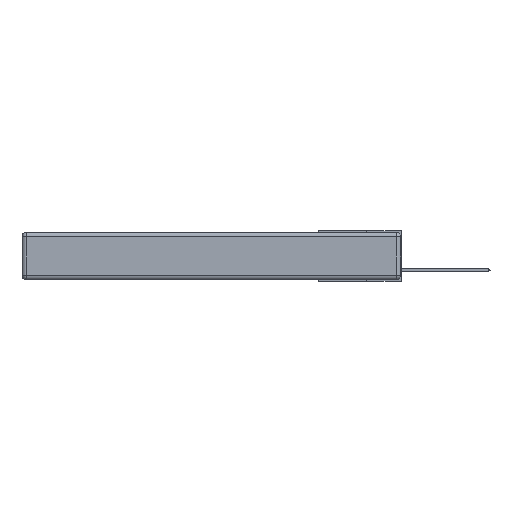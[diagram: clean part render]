
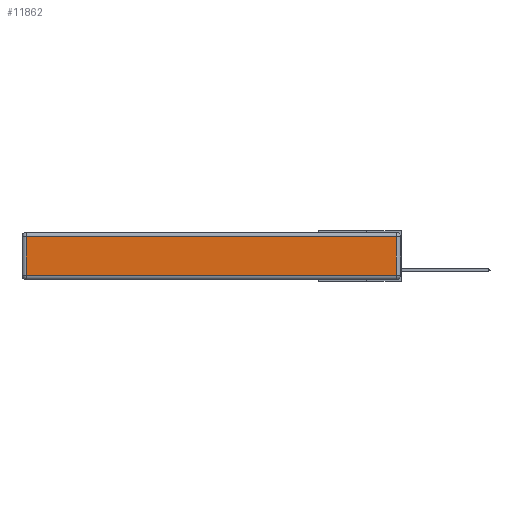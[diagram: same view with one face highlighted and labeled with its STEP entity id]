
A CAD part, left-side view. The second image highlights one B-rep face of the part: STEP entity #11862.
In plain terms, the highlighted planar face has unit normal (-1, 0, 0).
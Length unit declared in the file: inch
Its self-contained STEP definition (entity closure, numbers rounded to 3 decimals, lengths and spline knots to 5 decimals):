
#286 = CARTESIAN_POINT ( 'NONE',  ( 0., 2.72, -0.313 ) ) ;
#746 = CARTESIAN_POINT ( 'NONE',  ( 0., 0.03, -0.03 ) ) ;
#1514 = VECTOR ( 'NONE', #6466, 39.37008 ) ;
#2364 = VECTOR ( 'NONE', #9813, 39.37008 ) ;
#2687 = EDGE_LOOP ( 'NONE', ( #6443, #10497, #12969, #7129 ) ) ;
#3791 = CARTESIAN_POINT ( 'NONE',  ( 0., 2.72, -0.03 ) ) ;
#4362 = VERTEX_POINT ( 'NONE', #12095 ) ;
#4506 = VERTEX_POINT ( 'NONE', #746 ) ;
#5683 = VECTOR ( 'NONE', #15182, 39.37008 ) ;
#6097 = VERTEX_POINT ( 'NONE', #3791 ) ;
#6443 = ORIENTED_EDGE ( 'NONE', *, *, #14283, .T. ) ;
#6466 = DIRECTION ( 'NONE',  ( 0., 0., -1. ) ) ;
#6933 = LINE ( 'NONE', #11132, #1514 ) ;
#7129 = ORIENTED_EDGE ( 'NONE', *, *, #14841, .T. ) ;
#7217 = LINE ( 'NONE', #14725, #2364 ) ;
#9060 = LINE ( 'NONE', #11783, #10564 ) ;
#9475 = DIRECTION ( 'NONE',  ( 0., 0., 1. ) ) ;
#9650 = EDGE_CURVE ( 'NONE', #4506, #6097, #7217, .T. ) ;
#9813 = DIRECTION ( 'NONE',  ( 0., 1., 0. ) ) ;
#10497 = ORIENTED_EDGE ( 'NONE', *, *, #11649, .T. ) ;
#10564 = VECTOR ( 'NONE', #14358, 39.37008 ) ;
#10593 = CARTESIAN_POINT ( 'NONE',  ( 0., 0., -0.343 ) ) ;
#11132 = CARTESIAN_POINT ( 'NONE',  ( 0., 2.72, -0.343 ) ) ;
#11649 = EDGE_CURVE ( 'NONE', #4362, #4506, #13032, .T. ) ;
#11700 = CARTESIAN_POINT ( 'NONE',  ( 0., 0.03, -0.343 ) ) ;
#11783 = CARTESIAN_POINT ( 'NONE',  ( 0., 0., -0.313 ) ) ;
#11862 = ADVANCED_FACE ( 'NONE', ( #15291 ), #13162, .T. ) ;
#12095 = CARTESIAN_POINT ( 'NONE',  ( 0., 0.03, -0.313 ) ) ;
#12969 = ORIENTED_EDGE ( 'NONE', *, *, #9650, .T. ) ;
#13005 = DIRECTION ( 'NONE',  ( -1., 0., 0. ) ) ;
#13032 = LINE ( 'NONE', #11700, #5683 ) ;
#13162 = PLANE ( 'NONE',  #14309 ) ;
#13283 = VERTEX_POINT ( 'NONE', #286 ) ;
#14283 = EDGE_CURVE ( 'NONE', #13283, #4362, #9060, .T. ) ;
#14309 = AXIS2_PLACEMENT_3D ( 'NONE', #10593, #13005, #9475 ) ;
#14358 = DIRECTION ( 'NONE',  ( 0., -1., 0. ) ) ;
#14725 = CARTESIAN_POINT ( 'NONE',  ( 0., 2.75, -0.03 ) ) ;
#14841 = EDGE_CURVE ( 'NONE', #6097, #13283, #6933, .T. ) ;
#15182 = DIRECTION ( 'NONE',  ( 0., 0., 1. ) ) ;
#15291 = FACE_OUTER_BOUND ( 'NONE', #2687, .T. ) ;
